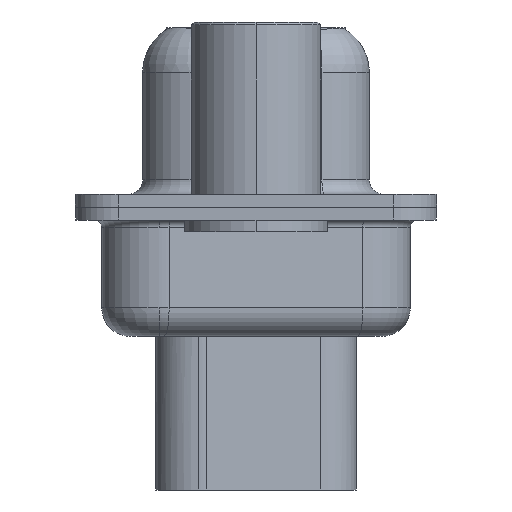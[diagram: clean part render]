
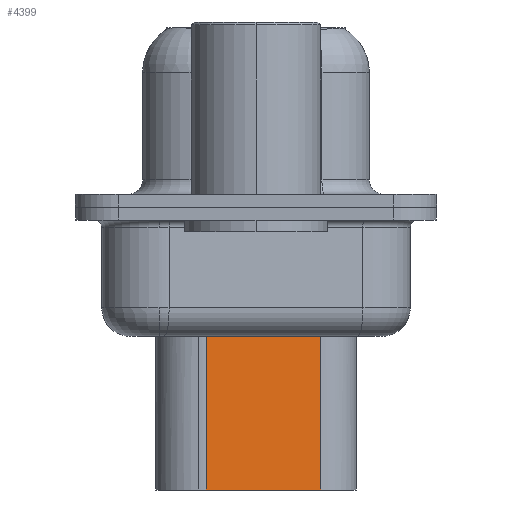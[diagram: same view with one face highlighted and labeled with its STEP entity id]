
A CAD part, left-side view. The second image highlights one B-rep face of the part: STEP entity #4399.
In plain terms, the highlighted planar face has unit normal (-0.985, -0.174, 0).
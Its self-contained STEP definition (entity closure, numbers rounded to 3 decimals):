
#775 = EDGE_LOOP ( 'NONE', ( #17670, #11838, #11616, #8062 ) ) ;
#1082 = VERTEX_POINT ( 'NONE', #14647 ) ;
#2782 = DIRECTION ( 'NONE',  ( -0.985, -0.174, 0. ) ) ;
#3553 = LINE ( 'NONE', #9380, #4445 ) ;
#3766 = VERTEX_POINT ( 'NONE', #12282 ) ;
#4078 = DIRECTION ( 'NONE',  ( 0., 0., -1. ) ) ;
#4399 = ADVANCED_FACE ( 'NONE', ( #7422 ), #7623, .T. ) ;
#4445 = VECTOR ( 'NONE', #9580, 1000. ) ;
#5327 = VERTEX_POINT ( 'NONE', #7465 ) ;
#5459 = LINE ( 'NONE', #13065, #9889 ) ;
#5697 = EDGE_CURVE ( 'NONE', #3766, #6029, #9030, .T. ) ;
#6029 = VERTEX_POINT ( 'NONE', #8671 ) ;
#7422 = FACE_OUTER_BOUND ( 'NONE', #775, .T. ) ;
#7465 = CARTESIAN_POINT ( 'NONE',  ( 5.214, -2.26, -9.85 ) ) ;
#7502 = DIRECTION ( 'NONE',  ( -0.174, 0.985, 0. ) ) ;
#7623 = PLANE ( 'NONE',  #19216 ) ;
#7939 = CARTESIAN_POINT ( 'NONE',  ( 4.338, 2.709, -3.975 ) ) ;
#8062 = ORIENTED_EDGE ( 'NONE', *, *, #17151, .F. ) ;
#8671 = CARTESIAN_POINT ( 'NONE',  ( 4.509, 1.74, -3.975 ) ) ;
#9008 = CARTESIAN_POINT ( 'NONE',  ( 4.509, 1.74, -3.1 ) ) ;
#9030 = LINE ( 'NONE', #7939, #15153 ) ;
#9380 = CARTESIAN_POINT ( 'NONE',  ( 5.214, -2.26, -3.1 ) ) ;
#9580 = DIRECTION ( 'NONE',  ( 0., 0., -1. ) ) ;
#9889 = VECTOR ( 'NONE', #4078, 1000. ) ;
#11574 = EDGE_CURVE ( 'NONE', #6029, #1082, #5459, .T. ) ;
#11616 = ORIENTED_EDGE ( 'NONE', *, *, #11574, .T. ) ;
#11757 = LINE ( 'NONE', #19576, #15149 ) ;
#11838 = ORIENTED_EDGE ( 'NONE', *, *, #5697, .T. ) ;
#12282 = CARTESIAN_POINT ( 'NONE',  ( 5.214, -2.26, -3.975 ) ) ;
#13065 = CARTESIAN_POINT ( 'NONE',  ( 4.509, 1.74, -3.1 ) ) ;
#14647 = CARTESIAN_POINT ( 'NONE',  ( 4.509, 1.74, -9.85 ) ) ;
#15149 = VECTOR ( 'NONE', #7502, 1000. ) ;
#15153 = VECTOR ( 'NONE', #18510, 1000. ) ;
#17151 = EDGE_CURVE ( 'NONE', #5327, #1082, #11757, .T. ) ;
#17328 = EDGE_CURVE ( 'NONE', #3766, #5327, #3553, .T. ) ;
#17670 = ORIENTED_EDGE ( 'NONE', *, *, #17328, .F. ) ;
#18510 = DIRECTION ( 'NONE',  ( -0.174, 0.985, 0. ) ) ;
#19216 = AXIS2_PLACEMENT_3D ( 'NONE', #9008, #2782, #19293 ) ;
#19293 = DIRECTION ( 'NONE',  ( 0.174, -0.985, 0. ) ) ;
#19576 = CARTESIAN_POINT ( 'NONE',  ( 4.509, 1.74, -9.85 ) ) ;
